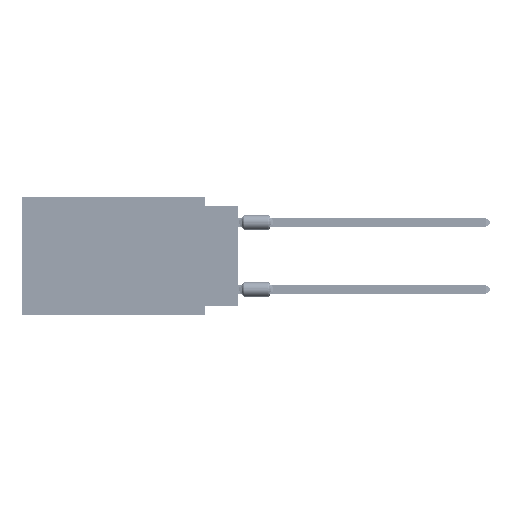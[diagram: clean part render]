
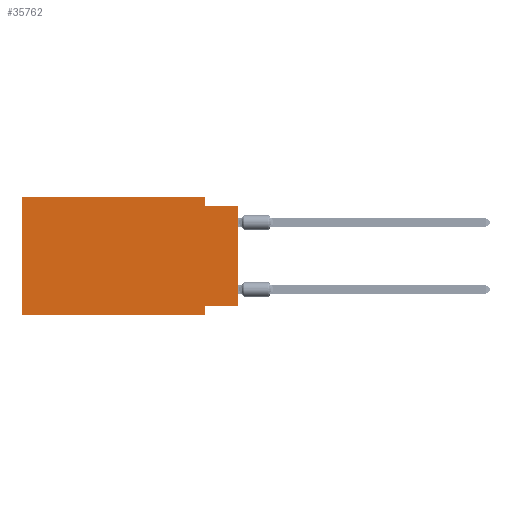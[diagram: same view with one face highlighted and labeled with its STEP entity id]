
A CAD part, left-side view. The second image highlights one B-rep face of the part: STEP entity #35762.
In plain terms, the highlighted planar face has unit normal (-1, 0, 0).
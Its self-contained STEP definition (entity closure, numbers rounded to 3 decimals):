
#158 = CARTESIAN_POINT ( 'NONE',  ( 0., 16.383, -8.89 ) ) ;
#236 = LINE ( 'NONE', #87221, #84852 ) ;
#936 = VERTEX_POINT ( 'NONE', #68603 ) ;
#7869 = DIRECTION ( 'NONE',  ( 0., 1., 0. ) ) ;
#8816 = VERTEX_POINT ( 'NONE', #46747 ) ;
#9723 = VECTOR ( 'NONE', #50670, 1000. ) ;
#14758 = EDGE_CURVE ( 'NONE', #21359, #38003, #77782, .T. ) ;
#15744 = LINE ( 'NONE', #35716, #37963 ) ;
#21049 = EDGE_CURVE ( 'NONE', #64054, #58665, #15744, .T. ) ;
#21359 = VERTEX_POINT ( 'NONE', #158 ) ;
#21378 = ORIENTED_EDGE ( 'NONE', *, *, #14758, .T. ) ;
#21647 = EDGE_CURVE ( 'NONE', #21359, #8816, #64433, .T. ) ;
#23356 = VECTOR ( 'NONE', #32741, 1000. ) ;
#24515 = ORIENTED_EDGE ( 'NONE', *, *, #45505, .F. ) ;
#27502 = EDGE_CURVE ( 'NONE', #87481, #38003, #70497, .T. ) ;
#28369 = FACE_OUTER_BOUND ( 'NONE', #49509, .T. ) ;
#31588 = CARTESIAN_POINT ( 'NONE',  ( 0., 16.383, -8.89 ) ) ;
#32741 = DIRECTION ( 'NONE',  ( 0., -1., 0. ) ) ;
#35716 = CARTESIAN_POINT ( 'NONE',  ( 0., 0., 0. ) ) ;
#35762 = ADVANCED_FACE ( 'NONE', ( #28369 ), #63400, .F. ) ;
#36308 = DIRECTION ( 'NONE',  ( 0., 0., -1. ) ) ;
#37247 = VECTOR ( 'NONE', #64456, 1000. ) ;
#37963 = VECTOR ( 'NONE', #49910, 1000. ) ;
#38003 = VERTEX_POINT ( 'NONE', #77836 ) ;
#39703 = EDGE_CURVE ( 'NONE', #936, #58665, #57292, .T. ) ;
#39847 = VECTOR ( 'NONE', #77718, 1000. ) ;
#40310 = EDGE_CURVE ( 'NONE', #64054, #87481, #68247, .T. ) ;
#43106 = CARTESIAN_POINT ( 'NONE',  ( 0., 0., -0.635 ) ) ;
#43195 = CARTESIAN_POINT ( 'NONE',  ( 0., 2.54, 0. ) ) ;
#45505 = EDGE_CURVE ( 'NONE', #8816, #53038, #53153, .T. ) ;
#46747 = CARTESIAN_POINT ( 'NONE',  ( 0., 16.383, 0. ) ) ;
#48771 = CARTESIAN_POINT ( 'NONE',  ( 0., 16.383, 0. ) ) ;
#49284 = ORIENTED_EDGE ( 'NONE', *, *, #54055, .F. ) ;
#49509 = EDGE_LOOP ( 'NONE', ( #80317, #77675, #49284, #24515, #69609, #21378, #79319, #85176 ) ) ;
#49910 = DIRECTION ( 'NONE',  ( 0., 0., 1. ) ) ;
#50670 = DIRECTION ( 'NONE',  ( 0., 0., 1. ) ) ;
#53038 = VERTEX_POINT ( 'NONE', #43195 ) ;
#53153 = LINE ( 'NONE', #65153, #23356 ) ;
#54055 = EDGE_CURVE ( 'NONE', #53038, #936, #236, .T. ) ;
#55006 = DIRECTION ( 'NONE',  ( 1., 0., 0. ) ) ;
#57292 = LINE ( 'NONE', #43106, #39847 ) ;
#57583 = DIRECTION ( 'NONE',  ( 0., 0., -1. ) ) ;
#58665 = VERTEX_POINT ( 'NONE', #62716 ) ;
#61044 = DIRECTION ( 'NONE',  ( 0., 0., -1. ) ) ;
#62454 = CARTESIAN_POINT ( 'NONE',  ( 0., 0., -8.255 ) ) ;
#62716 = CARTESIAN_POINT ( 'NONE',  ( 0., 0., -0.635 ) ) ;
#63400 = PLANE ( 'NONE',  #75302 ) ;
#64054 = VERTEX_POINT ( 'NONE', #71292 ) ;
#64433 = LINE ( 'NONE', #84399, #9723 ) ;
#64456 = DIRECTION ( 'NONE',  ( 0., -1., 0. ) ) ;
#65153 = CARTESIAN_POINT ( 'NONE',  ( 0., 16.383, 0. ) ) ;
#65436 = VECTOR ( 'NONE', #7869, 1000. ) ;
#68247 = LINE ( 'NONE', #62454, #65436 ) ;
#68603 = CARTESIAN_POINT ( 'NONE',  ( 0., 2.54, -0.635 ) ) ;
#69609 = ORIENTED_EDGE ( 'NONE', *, *, #21647, .F. ) ;
#69748 = VECTOR ( 'NONE', #57583, 1000. ) ;
#70068 = CARTESIAN_POINT ( 'NONE',  ( 0., 2.54, -8.89 ) ) ;
#70497 = LINE ( 'NONE', #70068, #69748 ) ;
#71292 = CARTESIAN_POINT ( 'NONE',  ( 0., 0., -8.255 ) ) ;
#75302 = AXIS2_PLACEMENT_3D ( 'NONE', #48771, #55006, #36308 ) ;
#77675 = ORIENTED_EDGE ( 'NONE', *, *, #39703, .F. ) ;
#77718 = DIRECTION ( 'NONE',  ( 0., -1., 0. ) ) ;
#77782 = LINE ( 'NONE', #31588, #37247 ) ;
#77836 = CARTESIAN_POINT ( 'NONE',  ( 0., 2.54, -8.89 ) ) ;
#79319 = ORIENTED_EDGE ( 'NONE', *, *, #27502, .F. ) ;
#80317 = ORIENTED_EDGE ( 'NONE', *, *, #21049, .T. ) ;
#81560 = CARTESIAN_POINT ( 'NONE',  ( 0., 2.54, -8.255 ) ) ;
#84399 = CARTESIAN_POINT ( 'NONE',  ( 0., 16.383, 0. ) ) ;
#84852 = VECTOR ( 'NONE', #61044, 1000. ) ;
#85176 = ORIENTED_EDGE ( 'NONE', *, *, #40310, .F. ) ;
#87221 = CARTESIAN_POINT ( 'NONE',  ( 0., 2.54, 0. ) ) ;
#87481 = VERTEX_POINT ( 'NONE', #81560 ) ;
